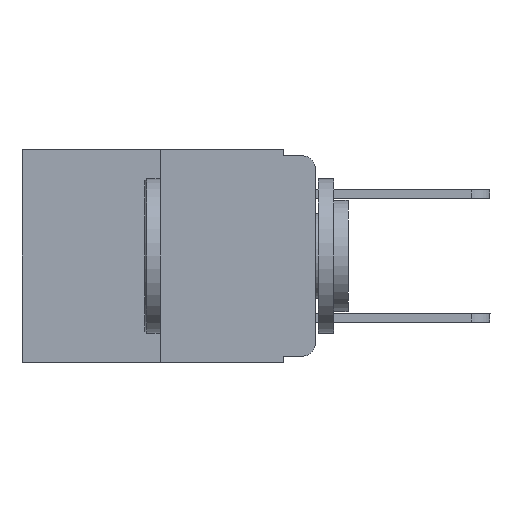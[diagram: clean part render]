
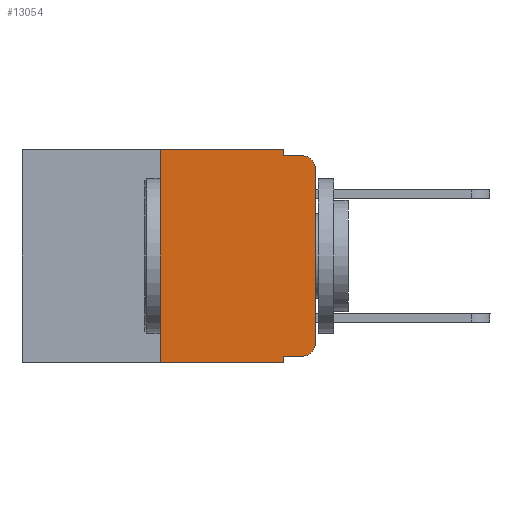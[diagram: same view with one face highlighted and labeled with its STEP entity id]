
A CAD part, left-side view. The second image highlights one B-rep face of the part: STEP entity #13054.
In plain terms, the highlighted planar face has unit normal (-1, 0, 0).
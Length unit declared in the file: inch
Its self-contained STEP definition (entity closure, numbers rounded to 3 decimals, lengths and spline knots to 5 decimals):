
#84 = DIRECTION ( 'NONE',  ( -1., 0., 0. ) ) ;
#353 = VECTOR ( 'NONE', #9768, 39.37008 ) ;
#1010 = VERTEX_POINT ( 'NONE', #9356 ) ;
#1234 = ORIENTED_EDGE ( 'NONE', *, *, #5261, .F. ) ;
#1264 = DIRECTION ( 'NONE',  ( 0., -1., 0. ) ) ;
#1653 = CARTESIAN_POINT ( 'NONE',  ( 0., 0.051, 0. ) ) ;
#1772 = EDGE_CURVE ( 'NONE', #4630, #6494, #2838, .T. ) ;
#1942 = CARTESIAN_POINT ( 'NONE',  ( 0., 0.25, 0. ) ) ;
#2178 = CARTESIAN_POINT ( 'NONE',  ( 0., 0.051, -0.333 ) ) ;
#2241 = CARTESIAN_POINT ( 'NONE',  ( 0., 0.051, -0.333 ) ) ;
#2701 = VECTOR ( 'NONE', #15485, 39.37008 ) ;
#2838 = CIRCLE ( 'NONE', #5587, 0.02 ) ;
#3677 = DIRECTION ( 'NONE',  ( 0., 0., -1. ) ) ;
#3971 = EDGE_CURVE ( 'NONE', #15219, #4630, #6725, .T. ) ;
#4112 = EDGE_LOOP ( 'NONE', ( #13621, #19374, #1234, #17204, #7253, #11351, #12922, #20017, #14870, #11654 ) ) ;
#4162 = CARTESIAN_POINT ( 'NONE',  ( 0., 0.473, -0.343 ) ) ;
#4630 = VERTEX_POINT ( 'NONE', #13572 ) ;
#5016 = VERTEX_POINT ( 'NONE', #9210 ) ;
#5261 = EDGE_CURVE ( 'NONE', #13729, #5016, #13666, .T. ) ;
#5399 = DIRECTION ( 'NONE',  ( 0., -1., 0. ) ) ;
#5533 = CARTESIAN_POINT ( 'NONE',  ( 0., 0.051, 0. ) ) ;
#5561 = CARTESIAN_POINT ( 'NONE',  ( 0., 0., 0. ) ) ;
#5587 = AXIS2_PLACEMENT_3D ( 'NONE', #15322, #84, #9163 ) ;
#5592 = EDGE_CURVE ( 'NONE', #17759, #18999, #13138, .T. ) ;
#5664 = CARTESIAN_POINT ( 'NONE',  ( 0., 0.051, -0.01 ) ) ;
#6494 = VERTEX_POINT ( 'NONE', #9930 ) ;
#6725 = LINE ( 'NONE', #2241, #9381 ) ;
#6790 = CARTESIAN_POINT ( 'NONE',  ( 0., 0.051, -0.01 ) ) ;
#7144 = DIRECTION ( 'NONE',  ( -1., 0., 0. ) ) ;
#7148 = PLANE ( 'NONE',  #18920 ) ;
#7253 = ORIENTED_EDGE ( 'NONE', *, *, #14081, .F. ) ;
#7435 = VERTEX_POINT ( 'NONE', #1653 ) ;
#8020 = CARTESIAN_POINT ( 'NONE',  ( 0., 0.051, 0. ) ) ;
#8572 = DIRECTION ( 'NONE',  ( 0., 0., -1. ) ) ;
#8681 = CARTESIAN_POINT ( 'NONE',  ( 0., 0.25, 0. ) ) ;
#8847 = DIRECTION ( 'NONE',  ( 1., 0., 0. ) ) ;
#9163 = DIRECTION ( 'NONE',  ( 0., 0., -1. ) ) ;
#9210 = CARTESIAN_POINT ( 'NONE',  ( 0., 0.02, -0.01 ) ) ;
#9321 = VECTOR ( 'NONE', #14844, 39.37008 ) ;
#9356 = CARTESIAN_POINT ( 'NONE',  ( 0., 0.051, -0.343 ) ) ;
#9381 = VECTOR ( 'NONE', #5399, 39.37008 ) ;
#9768 = DIRECTION ( 'NONE',  ( 0., 0., -1. ) ) ;
#9930 = CARTESIAN_POINT ( 'NONE',  ( 0., 0., -0.313 ) ) ;
#10194 = FACE_OUTER_BOUND ( 'NONE', #4112, .T. ) ;
#10389 = DIRECTION ( 'NONE',  ( 0., 0., -1. ) ) ;
#10711 = LINE ( 'NONE', #5561, #16044 ) ;
#10965 = EDGE_CURVE ( 'NONE', #7435, #13729, #12636, .T. ) ;
#11351 = ORIENTED_EDGE ( 'NONE', *, *, #5592, .F. ) ;
#11359 = EDGE_CURVE ( 'NONE', #15431, #5016, #12852, .T. ) ;
#11433 = CARTESIAN_POINT ( 'NONE',  ( 0., 0.25, -0.343 ) ) ;
#11434 = CARTESIAN_POINT ( 'NONE',  ( 0., 0., -0.03 ) ) ;
#11484 = EDGE_CURVE ( 'NONE', #6494, #15431, #10711, .T. ) ;
#11494 = CARTESIAN_POINT ( 'NONE',  ( 0., 0.02, -0.03 ) ) ;
#11654 = ORIENTED_EDGE ( 'NONE', *, *, #1772, .T. ) ;
#12636 = LINE ( 'NONE', #8020, #353 ) ;
#12852 = CIRCLE ( 'NONE', #13861, 0.02 ) ;
#12922 = ORIENTED_EDGE ( 'NONE', *, *, #14762, .T. ) ;
#13054 = ADVANCED_FACE ( 'NONE', ( #10194 ), #7148, .F. ) ;
#13138 = LINE ( 'NONE', #8681, #14609 ) ;
#13482 = LINE ( 'NONE', #5533, #19063 ) ;
#13510 = DIRECTION ( 'NONE',  ( 0., 0., 1. ) ) ;
#13572 = CARTESIAN_POINT ( 'NONE',  ( 0., 0.02, -0.333 ) ) ;
#13621 = ORIENTED_EDGE ( 'NONE', *, *, #11484, .T. ) ;
#13666 = LINE ( 'NONE', #5664, #9321 ) ;
#13729 = VERTEX_POINT ( 'NONE', #6790 ) ;
#13861 = AXIS2_PLACEMENT_3D ( 'NONE', #11494, #7144, #3677 ) ;
#14081 = EDGE_CURVE ( 'NONE', #18999, #7435, #17939, .T. ) ;
#14609 = VECTOR ( 'NONE', #13510, 39.37008 ) ;
#14748 = DIRECTION ( 'NONE',  ( 0., 0., 1. ) ) ;
#14762 = EDGE_CURVE ( 'NONE', #17759, #1010, #19930, .T. ) ;
#14844 = DIRECTION ( 'NONE',  ( 0., -1., 0. ) ) ;
#14854 = CARTESIAN_POINT ( 'NONE',  ( 0., 0.473, 0. ) ) ;
#14870 = ORIENTED_EDGE ( 'NONE', *, *, #3971, .T. ) ;
#15219 = VERTEX_POINT ( 'NONE', #2178 ) ;
#15322 = CARTESIAN_POINT ( 'NONE',  ( 0., 0.02, -0.313 ) ) ;
#15431 = VERTEX_POINT ( 'NONE', #11434 ) ;
#15485 = DIRECTION ( 'NONE',  ( 0., -1., 0. ) ) ;
#15807 = VECTOR ( 'NONE', #1264, 39.37008 ) ;
#16044 = VECTOR ( 'NONE', #14748, 39.37008 ) ;
#17204 = ORIENTED_EDGE ( 'NONE', *, *, #10965, .F. ) ;
#17759 = VERTEX_POINT ( 'NONE', #11433 ) ;
#17939 = LINE ( 'NONE', #18651, #2701 ) ;
#18651 = CARTESIAN_POINT ( 'NONE',  ( 0., 0.473, 0. ) ) ;
#18920 = AXIS2_PLACEMENT_3D ( 'NONE', #14854, #8847, #10389 ) ;
#18999 = VERTEX_POINT ( 'NONE', #1942 ) ;
#19063 = VECTOR ( 'NONE', #8572, 39.37008 ) ;
#19374 = ORIENTED_EDGE ( 'NONE', *, *, #11359, .T. ) ;
#19769 = EDGE_CURVE ( 'NONE', #15219, #1010, #13482, .T. ) ;
#19930 = LINE ( 'NONE', #4162, #15807 ) ;
#20017 = ORIENTED_EDGE ( 'NONE', *, *, #19769, .F. ) ;
